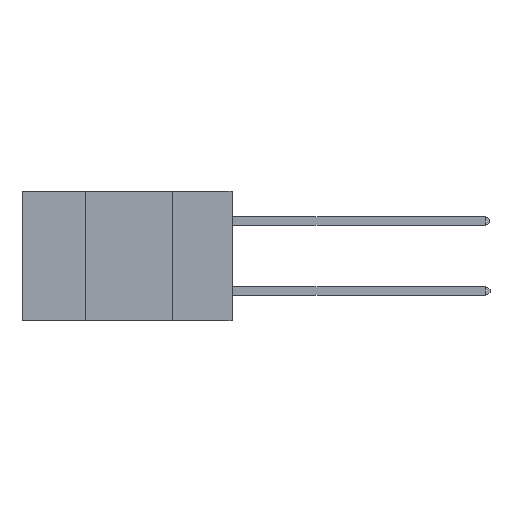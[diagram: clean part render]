
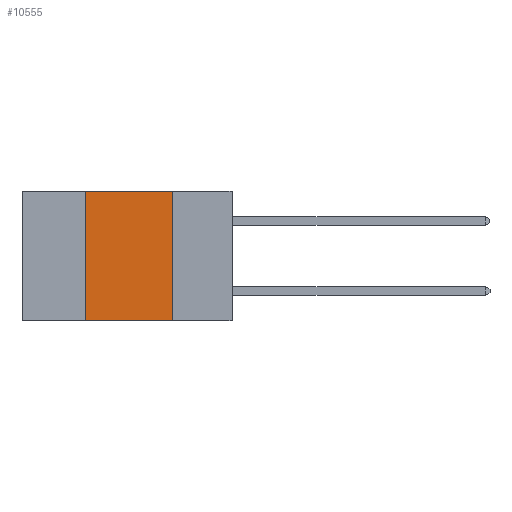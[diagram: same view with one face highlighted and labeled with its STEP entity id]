
A CAD part, left-side view. The second image highlights one B-rep face of the part: STEP entity #10555.
In plain terms, the highlighted planar face has unit normal (-1, 0, 0).
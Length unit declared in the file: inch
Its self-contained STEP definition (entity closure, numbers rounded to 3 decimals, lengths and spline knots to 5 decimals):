
#219 = CARTESIAN_POINT ( 'NONE',  ( 0., 0.6, -0.37 ) ) ;
#459 = VERTEX_POINT ( 'NONE', #8024 ) ;
#931 = CARTESIAN_POINT ( 'NONE',  ( 0., 0.17, 0. ) ) ;
#1846 = DIRECTION ( 'NONE',  ( 0., -1., 0. ) ) ;
#2613 = VERTEX_POINT ( 'NONE', #12169 ) ;
#2787 = EDGE_LOOP ( 'NONE', ( #9855, #9803, #14293, #9720 ) ) ;
#3149 = LINE ( 'NONE', #219, #14695 ) ;
#4114 = CARTESIAN_POINT ( 'NONE',  ( 0., 0.42, 0. ) ) ;
#4576 = DIRECTION ( 'NONE',  ( 0., 0., -1. ) ) ;
#5431 = EDGE_CURVE ( 'NONE', #2613, #16059, #5622, .T. ) ;
#5622 = LINE ( 'NONE', #931, #12852 ) ;
#5823 = CARTESIAN_POINT ( 'NONE',  ( 0., 0.17, -0.37 ) ) ;
#8024 = CARTESIAN_POINT ( 'NONE',  ( 0., 0.42, 0. ) ) ;
#8941 = CARTESIAN_POINT ( 'NONE',  ( 0., 0.6, 0. ) ) ;
#9114 = AXIS2_PLACEMENT_3D ( 'NONE', #8941, #13263, #4576 ) ;
#9265 = DIRECTION ( 'NONE',  ( 0., -1., 0. ) ) ;
#9700 = FACE_OUTER_BOUND ( 'NONE', #2787, .T. ) ;
#9720 = ORIENTED_EDGE ( 'NONE', *, *, #13559, .T. ) ;
#9803 = ORIENTED_EDGE ( 'NONE', *, *, #16916, .F. ) ;
#9855 = ORIENTED_EDGE ( 'NONE', *, *, #5431, .F. ) ;
#9900 = LINE ( 'NONE', #4114, #13676 ) ;
#10555 = ADVANCED_FACE ( 'NONE', ( #9700 ), #15942, .F. ) ;
#10619 = VERTEX_POINT ( 'NONE', #14767 ) ;
#11785 = LINE ( 'NONE', #13576, #15445 ) ;
#12169 = CARTESIAN_POINT ( 'NONE',  ( 0., 0.17, 0. ) ) ;
#12360 = EDGE_CURVE ( 'NONE', #10619, #459, #9900, .T. ) ;
#12844 = DIRECTION ( 'NONE',  ( 0., 0., 1. ) ) ;
#12852 = VECTOR ( 'NONE', #18173, 39.37008 ) ;
#13263 = DIRECTION ( 'NONE',  ( 1., 0., 0. ) ) ;
#13559 = EDGE_CURVE ( 'NONE', #10619, #16059, #3149, .T. ) ;
#13576 = CARTESIAN_POINT ( 'NONE',  ( 0., 0.6, 0. ) ) ;
#13676 = VECTOR ( 'NONE', #12844, 39.37008 ) ;
#14293 = ORIENTED_EDGE ( 'NONE', *, *, #12360, .F. ) ;
#14695 = VECTOR ( 'NONE', #9265, 39.37008 ) ;
#14767 = CARTESIAN_POINT ( 'NONE',  ( 0., 0.42, -0.37 ) ) ;
#15445 = VECTOR ( 'NONE', #1846, 39.37008 ) ;
#15942 = PLANE ( 'NONE',  #9114 ) ;
#16059 = VERTEX_POINT ( 'NONE', #5823 ) ;
#16916 = EDGE_CURVE ( 'NONE', #459, #2613, #11785, .T. ) ;
#18173 = DIRECTION ( 'NONE',  ( 0., 0., -1. ) ) ;
